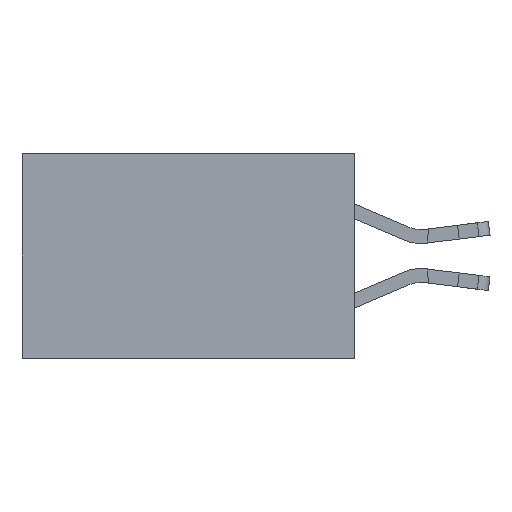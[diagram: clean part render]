
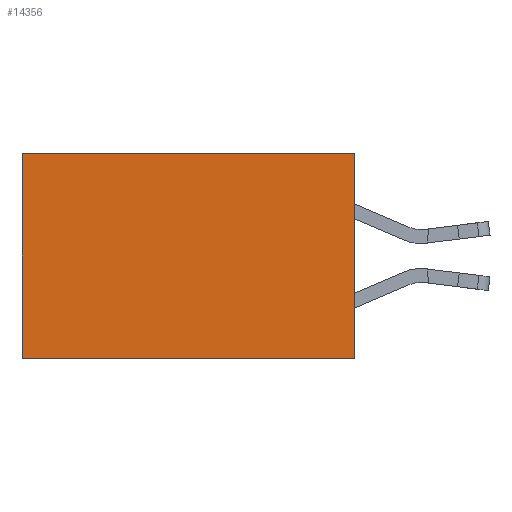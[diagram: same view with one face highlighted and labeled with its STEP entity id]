
A CAD part, left-side view. The second image highlights one B-rep face of the part: STEP entity #14356.
In plain terms, the highlighted planar face has unit normal (-1, 0, 0).
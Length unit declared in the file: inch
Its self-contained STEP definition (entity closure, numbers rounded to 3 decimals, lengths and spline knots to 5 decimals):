
#199 = VERTEX_POINT ( 'NONE', #6070 ) ;
#869 = VECTOR ( 'NONE', #14720, 39.37008 ) ;
#1265 = EDGE_CURVE ( 'NONE', #17213, #9077, #2002, .T. ) ;
#1441 = ORIENTED_EDGE ( 'NONE', *, *, #1265, .F. ) ;
#1812 = DIRECTION ( 'NONE',  ( 0., 0., -1. ) ) ;
#1843 = DIRECTION ( 'NONE',  ( 1., 0., 0. ) ) ;
#1976 = PLANE ( 'NONE',  #15500 ) ;
#2002 = LINE ( 'NONE', #5769, #15772 ) ;
#2103 = CARTESIAN_POINT ( 'NONE',  ( 0.298, 0., 0. ) ) ;
#3018 = DIRECTION ( 'NONE',  ( 0., 0., -1. ) ) ;
#3864 = CARTESIAN_POINT ( 'NONE',  ( 0.298, 0., -0.37 ) ) ;
#4056 = VERTEX_POINT ( 'NONE', #13327 ) ;
#4733 = CARTESIAN_POINT ( 'NONE',  ( 0.298, 0.6, 0. ) ) ;
#4862 = DIRECTION ( 'NONE',  ( 0., 0., -1. ) ) ;
#5052 = EDGE_CURVE ( 'NONE', #9077, #199, #7480, .T. ) ;
#5769 = CARTESIAN_POINT ( 'NONE',  ( 0.298, 0., 0. ) ) ;
#6070 = CARTESIAN_POINT ( 'NONE',  ( 0.298, 0.6, -0.37 ) ) ;
#7126 = LINE ( 'NONE', #15598, #11226 ) ;
#7480 = LINE ( 'NONE', #11601, #869 ) ;
#8437 = EDGE_CURVE ( 'NONE', #17213, #4056, #7126, .T. ) ;
#8991 = EDGE_CURVE ( 'NONE', #4056, #199, #11657, .T. ) ;
#9077 = VERTEX_POINT ( 'NONE', #3864 ) ;
#11226 = VECTOR ( 'NONE', #15558, 39.37008 ) ;
#11440 = ORIENTED_EDGE ( 'NONE', *, *, #5052, .F. ) ;
#11447 = EDGE_LOOP ( 'NONE', ( #12536, #11440, #1441, #12628 ) ) ;
#11601 = CARTESIAN_POINT ( 'NONE',  ( 0.298, 0., -0.37 ) ) ;
#11657 = LINE ( 'NONE', #4733, #14836 ) ;
#12536 = ORIENTED_EDGE ( 'NONE', *, *, #8991, .T. ) ;
#12628 = ORIENTED_EDGE ( 'NONE', *, *, #8437, .T. ) ;
#12745 = CARTESIAN_POINT ( 'NONE',  ( 0.298, 0., 0. ) ) ;
#13327 = CARTESIAN_POINT ( 'NONE',  ( 0.298, 0.6, 0. ) ) ;
#13639 = FACE_OUTER_BOUND ( 'NONE', #11447, .T. ) ;
#14356 = ADVANCED_FACE ( 'NONE', ( #13639 ), #1976, .F. ) ;
#14720 = DIRECTION ( 'NONE',  ( 0., 1., 0. ) ) ;
#14836 = VECTOR ( 'NONE', #3018, 39.37008 ) ;
#15500 = AXIS2_PLACEMENT_3D ( 'NONE', #2103, #1843, #1812 ) ;
#15558 = DIRECTION ( 'NONE',  ( 0., 1., 0. ) ) ;
#15598 = CARTESIAN_POINT ( 'NONE',  ( 0.298, 0., 0. ) ) ;
#15772 = VECTOR ( 'NONE', #4862, 39.37008 ) ;
#17213 = VERTEX_POINT ( 'NONE', #12745 ) ;
